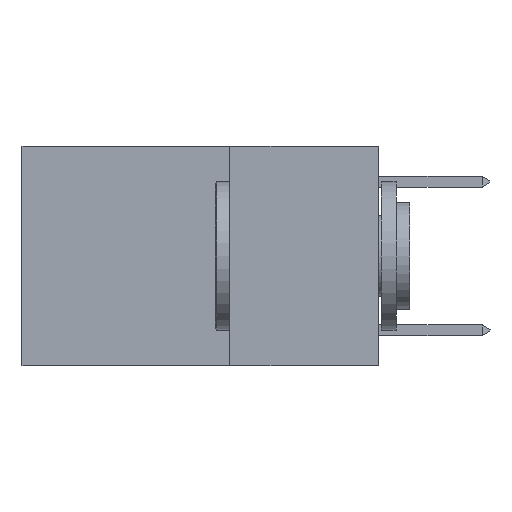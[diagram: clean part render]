
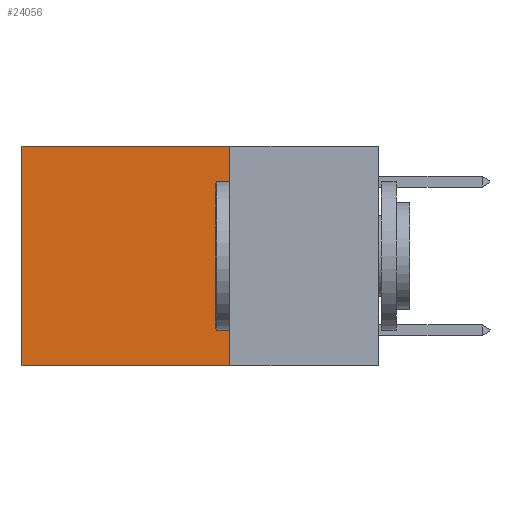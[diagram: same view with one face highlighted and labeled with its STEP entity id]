
A CAD part, left-side view. The second image highlights one B-rep face of the part: STEP entity #24056.
In plain terms, the highlighted planar face has unit normal (-1, 0, 0).
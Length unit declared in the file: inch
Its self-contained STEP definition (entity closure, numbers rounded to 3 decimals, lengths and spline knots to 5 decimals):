
#448 = DIRECTION ( 'NONE',  ( 0., 0., -1. ) ) ;
#727 = AXIS2_PLACEMENT_3D ( 'NONE', #26516, #11834, #28901 ) ;
#1683 = PLANE ( 'NONE',  #727 ) ;
#2845 = VERTEX_POINT ( 'NONE', #19505 ) ;
#3099 = EDGE_CURVE ( 'NONE', #5020, #15209, #31795, .T. ) ;
#3331 = ORIENTED_EDGE ( 'NONE', *, *, #3099, .T. ) ;
#3511 = CARTESIAN_POINT ( 'NONE',  ( 0.2625, 0.6, 0. ) ) ;
#4308 = CARTESIAN_POINT ( 'NONE',  ( 0.2625, 0.25, 0. ) ) ;
#4574 = ORIENTED_EDGE ( 'NONE', *, *, #29672, .F. ) ;
#5020 = VERTEX_POINT ( 'NONE', #3511 ) ;
#6739 = EDGE_LOOP ( 'NONE', ( #3331, #4574, #9452, #7553 ) ) ;
#6867 = DIRECTION ( 'NONE',  ( 0., 0., -1. ) ) ;
#7553 = ORIENTED_EDGE ( 'NONE', *, *, #27570, .T. ) ;
#9452 = ORIENTED_EDGE ( 'NONE', *, *, #22002, .F. ) ;
#11834 = DIRECTION ( 'NONE',  ( 1., 0., 0. ) ) ;
#12351 = DIRECTION ( 'NONE',  ( 0., 1., 0. ) ) ;
#13120 = VECTOR ( 'NONE', #28144, 39.37008 ) ;
#13588 = CARTESIAN_POINT ( 'NONE',  ( 0.2625, 0.25, 0. ) ) ;
#13794 = VECTOR ( 'NONE', #448, 39.37008 ) ;
#15209 = VERTEX_POINT ( 'NONE', #30462 ) ;
#15455 = CARTESIAN_POINT ( 'NONE',  ( 0.2625, 0.6, 0. ) ) ;
#19050 = VECTOR ( 'NONE', #6867, 39.37008 ) ;
#19505 = CARTESIAN_POINT ( 'NONE',  ( 0.2625, 0.25, 0. ) ) ;
#19708 = LINE ( 'NONE', #13588, #13120 ) ;
#22002 = EDGE_CURVE ( 'NONE', #2845, #24039, #31788, .T. ) ;
#23389 = FACE_OUTER_BOUND ( 'NONE', #6739, .T. ) ;
#24039 = VERTEX_POINT ( 'NONE', #26411 ) ;
#24056 = ADVANCED_FACE ( 'NONE', ( #23389 ), #1683, .F. ) ;
#24174 = LINE ( 'NONE', #24727, #28285 ) ;
#24727 = CARTESIAN_POINT ( 'NONE',  ( 0.2625, 0.25, -0.37 ) ) ;
#26411 = CARTESIAN_POINT ( 'NONE',  ( 0.2625, 0.25, -0.37 ) ) ;
#26516 = CARTESIAN_POINT ( 'NONE',  ( 0.2625, 0.25, 0. ) ) ;
#27570 = EDGE_CURVE ( 'NONE', #2845, #5020, #19708, .T. ) ;
#28144 = DIRECTION ( 'NONE',  ( 0., 1., 0. ) ) ;
#28285 = VECTOR ( 'NONE', #12351, 39.37008 ) ;
#28901 = DIRECTION ( 'NONE',  ( 0., 0., -1. ) ) ;
#29672 = EDGE_CURVE ( 'NONE', #24039, #15209, #24174, .T. ) ;
#30462 = CARTESIAN_POINT ( 'NONE',  ( 0.2625, 0.6, -0.37 ) ) ;
#31788 = LINE ( 'NONE', #4308, #19050 ) ;
#31795 = LINE ( 'NONE', #15455, #13794 ) ;
